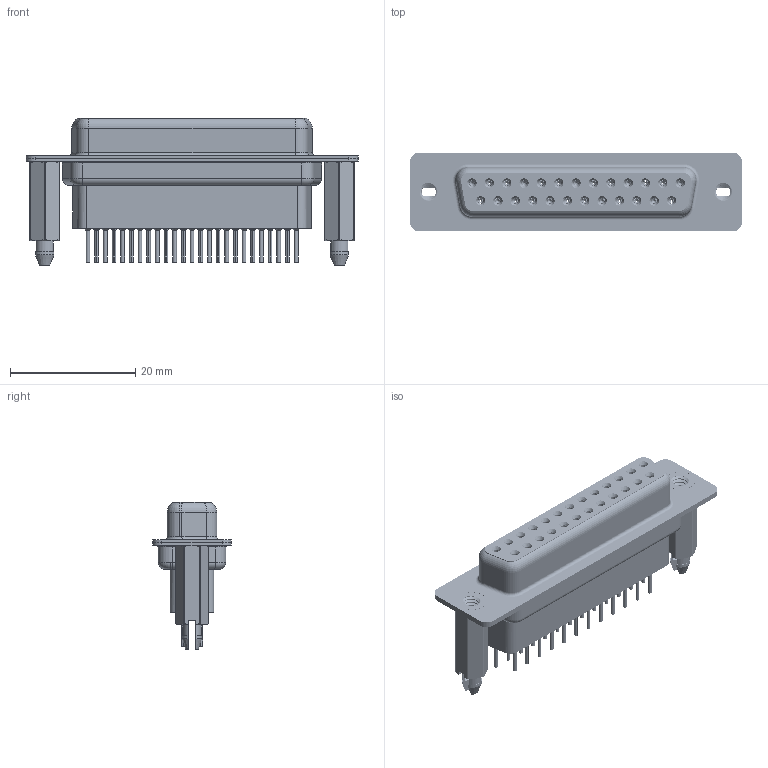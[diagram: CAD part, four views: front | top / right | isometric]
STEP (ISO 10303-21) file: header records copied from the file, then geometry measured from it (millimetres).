
FILE_DESCRIPTION (( 'STEP AP203' ), '1' );
FILE_NAME ('628-025-251-056.STEP', '2020-07-14T06:24:13', ( '' ), ( '' ), 'SwSTEP 2.0', 'SolidWorks 2020', '' );
FILE_SCHEMA (( 'CONFIG_CONTROL_DESIGN' ));
Length unit declared in the file: millimetre
Products named in the file (7): 628-025-251-056; 628 Shell Rear_25 Contacts; 628 Shell Front_25 Contacts; 628 Housing_25 HP; 628 4-40 Threaded Boardlock_HP51; 628 Contact Row 2_51; 628 Contact Row 1_51
Assembly tree (30 placements, depth 2):
  628-025-251-056
    628 Housing_25 HP
    628 Shell Front_25 Contacts
    628 Shell Rear_25 Contacts
    628 Contact Row 1_51  x13
    628 Contact Row 2_51  x12
    628 4-40 Threaded Boardlock_HP51  x2
Bounding box: 53 x 12.6 x 23.6 mm (x, y, z)
Volume: 5317 mm3; surface area: 12166.8 mm2
Topology: 30 solids, 30 shells, 3428 faces, 8817 edges, 5508 vertices
Faces by surface type: cylinder 994, plane 874, torus 663, bspline 506, cone 391
Entity records: 29002 total; most frequent: CARTESIAN_POINT 8064, DIRECTION 4280, ORIENTED_EDGE 3988, EDGE_CURVE 1994, AXIS2_PLACEMENT_3D 1781, VERTEX_POINT 1261, EDGE_LOOP 975, CIRCLE 963
